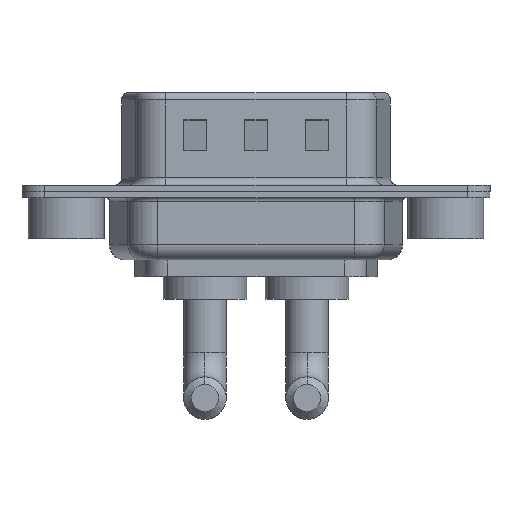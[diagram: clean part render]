
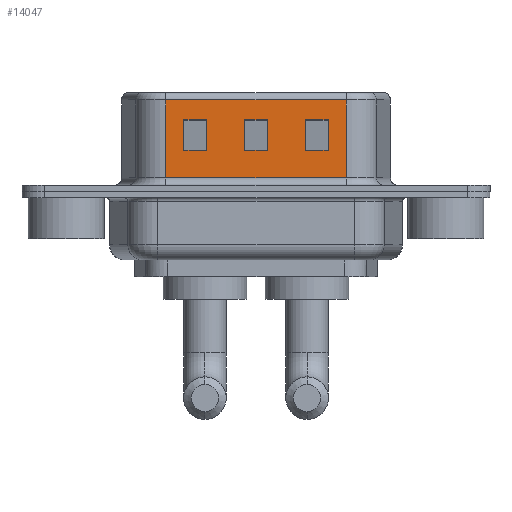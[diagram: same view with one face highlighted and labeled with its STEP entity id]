
A CAD part, front view. The second image highlights one B-rep face of the part: STEP entity #14047.
In plain terms, the highlighted planar face has unit normal (0, -1, 0).
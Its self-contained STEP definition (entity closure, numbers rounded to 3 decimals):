
#44 = EDGE_CURVE ( 'NONE', #1294, #1071, #5718, .T. ) ;
#108 = VECTOR ( 'NONE', #3685, 1000. ) ;
#197 = CARTESIAN_POINT ( 'NONE',  ( 18.451, -4.55, 4.705 ) ) ;
#276 = LINE ( 'NONE', #197, #7513 ) ;
#309 = VECTOR ( 'NONE', #13575, 1000. ) ;
#353 = EDGE_CURVE ( 'NONE', #12192, #2662, #3419, .T. ) ;
#361 = CARTESIAN_POINT ( 'NONE',  ( 6.549, -4.55, 6.52 ) ) ;
#423 = DIRECTION ( 'NONE',  ( 1., 0., 0. ) ) ;
#460 = VECTOR ( 'NONE', #11211, 1000. ) ;
#532 = CARTESIAN_POINT ( 'NONE',  ( 15.75, -4.55, 6.52 ) ) ;
#683 = EDGE_CURVE ( 'NONE', #10813, #12192, #4142, .T. ) ;
#692 = VERTEX_POINT ( 'NONE', #11877 ) ;
#767 = CARTESIAN_POINT ( 'NONE',  ( 17.25, -4.55, 4.705 ) ) ;
#826 = CARTESIAN_POINT ( 'NONE',  ( 18.451, -4.55, 2.705 ) ) ;
#1067 = LINE ( 'NONE', #3154, #5421 ) ;
#1071 = VERTEX_POINT ( 'NONE', #12216 ) ;
#1136 = EDGE_CURVE ( 'NONE', #8353, #10607, #5665, .T. ) ;
#1151 = VECTOR ( 'NONE', #1353, 1000. ) ;
#1194 = DIRECTION ( 'NONE',  ( 0., 0., -1. ) ) ;
#1294 = VERTEX_POINT ( 'NONE', #2602 ) ;
#1353 = DIRECTION ( 'NONE',  ( 1., 0., 0. ) ) ;
#1393 = DIRECTION ( 'NONE',  ( -1., 0., 0. ) ) ;
#1421 = LINE ( 'NONE', #9109, #309 ) ;
#1455 = DIRECTION ( 'NONE',  ( 0., 0., -1. ) ) ;
#1548 = LINE ( 'NONE', #532, #8897 ) ;
#1784 = CARTESIAN_POINT ( 'NONE',  ( 18.451, -4.55, 0.9 ) ) ;
#1899 = DIRECTION ( 'NONE',  ( 1., 0., 0. ) ) ;
#1976 = CARTESIAN_POINT ( 'NONE',  ( 18.451, -4.55, 6.52 ) ) ;
#2367 = CARTESIAN_POINT ( 'NONE',  ( 14.451, -4.55, 4.705 ) ) ;
#2430 = CARTESIAN_POINT ( 'NONE',  ( 7.75, -4.55, 4.705 ) ) ;
#2438 = EDGE_CURVE ( 'NONE', #2662, #14277, #276, .T. ) ;
#2602 = CARTESIAN_POINT ( 'NONE',  ( 17.25, -4.55, 2.705 ) ) ;
#2618 = FACE_BOUND ( 'NONE', #11335, .T. ) ;
#2644 = VECTOR ( 'NONE', #1899, 1000. ) ;
#2662 = VERTEX_POINT ( 'NONE', #13542 ) ;
#2696 = ORIENTED_EDGE ( 'NONE', *, *, #12803, .T. ) ;
#2699 = EDGE_CURVE ( 'NONE', #11807, #13393, #10158, .T. ) ;
#2701 = CARTESIAN_POINT ( 'NONE',  ( 22.451, -4.55, 4.705 ) ) ;
#2750 = DIRECTION ( 'NONE',  ( 0., 0., -1. ) ) ;
#3048 = CARTESIAN_POINT ( 'NONE',  ( 6.549, -4.55, 6.02 ) ) ;
#3091 = CARTESIAN_POINT ( 'NONE',  ( 6.549, -4.55, 0.9 ) ) ;
#3154 = CARTESIAN_POINT ( 'NONE',  ( 18.451, -4.55, 0.9 ) ) ;
#3283 = VERTEX_POINT ( 'NONE', #1784 ) ;
#3419 = LINE ( 'NONE', #9025, #460 ) ;
#3474 = LINE ( 'NONE', #13687, #13832 ) ;
#3685 = DIRECTION ( 'NONE',  ( -1., 0., 0. ) ) ;
#3700 = CARTESIAN_POINT ( 'NONE',  ( 18.451, -4.55, 6.52 ) ) ;
#3823 = ORIENTED_EDGE ( 'NONE', *, *, #7382, .F. ) ;
#4053 = CARTESIAN_POINT ( 'NONE',  ( 13.25, -4.55, 4.705 ) ) ;
#4122 = EDGE_CURVE ( 'NONE', #4925, #9214, #12835, .T. ) ;
#4142 = LINE ( 'NONE', #826, #13815 ) ;
#4289 = DIRECTION ( 'NONE',  ( 0., 0., -1. ) ) ;
#4372 = EDGE_LOOP ( 'NONE', ( #3823, #12500, #10245, #10065 ) ) ;
#4397 = CARTESIAN_POINT ( 'NONE',  ( 9.25, -4.55, 4.705 ) ) ;
#4514 = EDGE_CURVE ( 'NONE', #14277, #10813, #3474, .T. ) ;
#4555 = CARTESIAN_POINT ( 'NONE',  ( 7.75, -4.55, 6.52 ) ) ;
#4636 = VECTOR ( 'NONE', #13105, 1000. ) ;
#4819 = LINE ( 'NONE', #11378, #12392 ) ;
#4925 = VERTEX_POINT ( 'NONE', #12272 ) ;
#5077 = ORIENTED_EDGE ( 'NONE', *, *, #10925, .T. ) ;
#5421 = VECTOR ( 'NONE', #7449, 1000. ) ;
#5665 = LINE ( 'NONE', #4555, #4636 ) ;
#5718 = LINE ( 'NONE', #8175, #8540 ) ;
#5874 = DIRECTION ( 'NONE',  ( -1., 0., 0. ) ) ;
#6735 = VECTOR ( 'NONE', #4289, 1000. ) ;
#6880 = CARTESIAN_POINT ( 'NONE',  ( 9.25, -4.55, 2.705 ) ) ;
#7023 = ORIENTED_EDGE ( 'NONE', *, *, #1136, .T. ) ;
#7114 = LINE ( 'NONE', #9217, #108 ) ;
#7127 = FACE_BOUND ( 'NONE', #8555, .T. ) ;
#7209 = ORIENTED_EDGE ( 'NONE', *, *, #353, .T. ) ;
#7382 = EDGE_CURVE ( 'NONE', #692, #3283, #9528, .T. ) ;
#7449 = DIRECTION ( 'NONE',  ( 1., 0., 0. ) ) ;
#7485 = VECTOR ( 'NONE', #1455, 1000. ) ;
#7513 = VECTOR ( 'NONE', #423, 1000. ) ;
#7610 = CARTESIAN_POINT ( 'NONE',  ( 11.75, -4.55, 2.705 ) ) ;
#7892 = LINE ( 'NONE', #2367, #1151 ) ;
#7920 = DIRECTION ( 'NONE',  ( 0., 0., -1. ) ) ;
#7967 = EDGE_CURVE ( 'NONE', #13442, #10257, #11501, .T. ) ;
#8175 = CARTESIAN_POINT ( 'NONE',  ( 22.451, -4.55, 2.705 ) ) ;
#8353 = VERTEX_POINT ( 'NONE', #10226 ) ;
#8540 = VECTOR ( 'NONE', #5874, 1000. ) ;
#8555 = EDGE_LOOP ( 'NONE', ( #5077, #9543, #2696, #10145 ) ) ;
#8897 = VECTOR ( 'NONE', #9593, 1000. ) ;
#8942 = EDGE_CURVE ( 'NONE', #10607, #13442, #7892, .T. ) ;
#8985 = VECTOR ( 'NONE', #2750, 1000. ) ;
#9004 = DIRECTION ( 'NONE',  ( 0., 1., 0. ) ) ;
#9025 = CARTESIAN_POINT ( 'NONE',  ( 11.75, -4.55, 6.52 ) ) ;
#9109 = CARTESIAN_POINT ( 'NONE',  ( 18.451, -4.55, 6.02 ) ) ;
#9214 = VERTEX_POINT ( 'NONE', #767 ) ;
#9217 = CARTESIAN_POINT ( 'NONE',  ( 14.451, -4.55, 2.705 ) ) ;
#9230 = FACE_OUTER_BOUND ( 'NONE', #4372, .T. ) ;
#9528 = LINE ( 'NONE', #1976, #6735 ) ;
#9543 = ORIENTED_EDGE ( 'NONE', *, *, #44, .T. ) ;
#9593 = DIRECTION ( 'NONE',  ( 0., 0., 1. ) ) ;
#10065 = ORIENTED_EDGE ( 'NONE', *, *, #10558, .T. ) ;
#10145 = ORIENTED_EDGE ( 'NONE', *, *, #4122, .T. ) ;
#10158 = LINE ( 'NONE', #361, #7485 ) ;
#10226 = CARTESIAN_POINT ( 'NONE',  ( 7.75, -4.55, 2.705 ) ) ;
#10245 = ORIENTED_EDGE ( 'NONE', *, *, #2699, .T. ) ;
#10257 = VERTEX_POINT ( 'NONE', #6880 ) ;
#10389 = ORIENTED_EDGE ( 'NONE', *, *, #8942, .T. ) ;
#10558 = EDGE_CURVE ( 'NONE', #13393, #3283, #1067, .T. ) ;
#10602 = EDGE_CURVE ( 'NONE', #692, #11807, #1421, .T. ) ;
#10607 = VERTEX_POINT ( 'NONE', #2430 ) ;
#10813 = VERTEX_POINT ( 'NONE', #10950 ) ;
#10925 = EDGE_CURVE ( 'NONE', #9214, #1294, #4819, .T. ) ;
#10950 = CARTESIAN_POINT ( 'NONE',  ( 13.25, -4.55, 2.705 ) ) ;
#11211 = DIRECTION ( 'NONE',  ( 0., 0., 1. ) ) ;
#11335 = EDGE_LOOP ( 'NONE', ( #13042, #11761, #7023, #10389 ) ) ;
#11351 = FACE_BOUND ( 'NONE', #14257, .T. ) ;
#11378 = CARTESIAN_POINT ( 'NONE',  ( 17.25, -4.55, 6.52 ) ) ;
#11501 = LINE ( 'NONE', #13765, #8985 ) ;
#11761 = ORIENTED_EDGE ( 'NONE', *, *, #11998, .T. ) ;
#11807 = VERTEX_POINT ( 'NONE', #3048 ) ;
#11838 = AXIS2_PLACEMENT_3D ( 'NONE', #3700, #9004, #1393 ) ;
#11861 = ORIENTED_EDGE ( 'NONE', *, *, #4514, .T. ) ;
#11877 = CARTESIAN_POINT ( 'NONE',  ( 18.451, -4.55, 6.02 ) ) ;
#11998 = EDGE_CURVE ( 'NONE', #10257, #8353, #7114, .T. ) ;
#12192 = VERTEX_POINT ( 'NONE', #7610 ) ;
#12216 = CARTESIAN_POINT ( 'NONE',  ( 15.75, -4.55, 2.705 ) ) ;
#12272 = CARTESIAN_POINT ( 'NONE',  ( 15.75, -4.55, 4.705 ) ) ;
#12392 = VECTOR ( 'NONE', #1194, 1000. ) ;
#12454 = PLANE ( 'NONE',  #11838 ) ;
#12500 = ORIENTED_EDGE ( 'NONE', *, *, #10602, .T. ) ;
#12803 = EDGE_CURVE ( 'NONE', #1071, #4925, #1548, .T. ) ;
#12835 = LINE ( 'NONE', #2701, #2644 ) ;
#12972 = DIRECTION ( 'NONE',  ( -1., 0., 0. ) ) ;
#13006 = ORIENTED_EDGE ( 'NONE', *, *, #2438, .T. ) ;
#13042 = ORIENTED_EDGE ( 'NONE', *, *, #7967, .T. ) ;
#13105 = DIRECTION ( 'NONE',  ( 0., 0., 1. ) ) ;
#13393 = VERTEX_POINT ( 'NONE', #3091 ) ;
#13442 = VERTEX_POINT ( 'NONE', #4397 ) ;
#13542 = CARTESIAN_POINT ( 'NONE',  ( 11.75, -4.55, 4.705 ) ) ;
#13575 = DIRECTION ( 'NONE',  ( -1., 0., 0. ) ) ;
#13687 = CARTESIAN_POINT ( 'NONE',  ( 13.25, -4.55, 6.52 ) ) ;
#13765 = CARTESIAN_POINT ( 'NONE',  ( 9.25, -4.55, 6.52 ) ) ;
#13815 = VECTOR ( 'NONE', #12972, 1000. ) ;
#13832 = VECTOR ( 'NONE', #7920, 1000. ) ;
#14047 = ADVANCED_FACE ( 'NONE', ( #2618, #7127, #11351, #9230 ), #12454, .F. ) ;
#14192 = ORIENTED_EDGE ( 'NONE', *, *, #683, .T. ) ;
#14257 = EDGE_LOOP ( 'NONE', ( #13006, #11861, #14192, #7209 ) ) ;
#14277 = VERTEX_POINT ( 'NONE', #4053 ) ;
